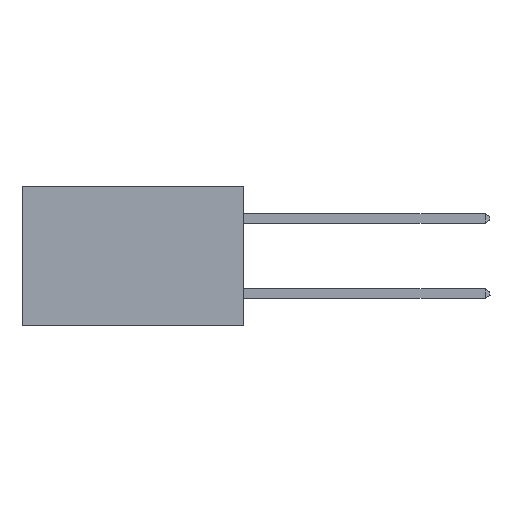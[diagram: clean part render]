
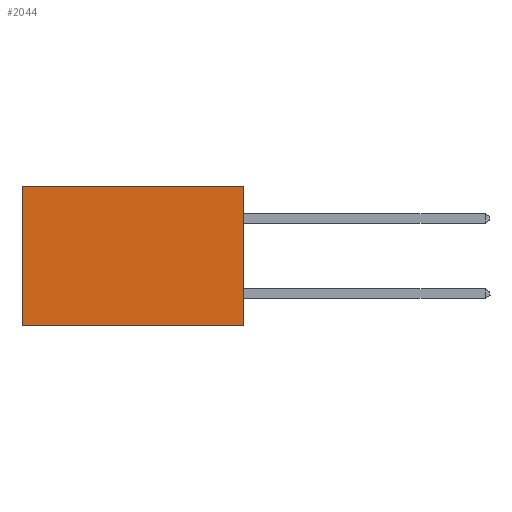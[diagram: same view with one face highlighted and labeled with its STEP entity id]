
A CAD part, left-side view. The second image highlights one B-rep face of the part: STEP entity #2044.
In plain terms, the highlighted planar face has unit normal (-1, 0, 0).
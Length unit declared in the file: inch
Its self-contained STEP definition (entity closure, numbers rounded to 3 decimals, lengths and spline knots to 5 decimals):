
#309 = CARTESIAN_POINT ( 'NONE',  ( 0.277, 0., 0. ) ) ;
#1711 = CARTESIAN_POINT ( 'NONE',  ( 0.277, 0.59, 0. ) ) ;
#2044 = ADVANCED_FACE ( 'NONE', ( #8573 ), #7231, .F. ) ;
#3269 = ORIENTED_EDGE ( 'NONE', *, *, #14440, .F. ) ;
#3280 = VERTEX_POINT ( 'NONE', #16151 ) ;
#4182 = VERTEX_POINT ( 'NONE', #17679 ) ;
#4478 = VECTOR ( 'NONE', #14712, 39.37008 ) ;
#4995 = EDGE_CURVE ( 'NONE', #7809, #6947, #7499, .T. ) ;
#6272 = LINE ( 'NONE', #16073, #9992 ) ;
#6947 = VERTEX_POINT ( 'NONE', #1711 ) ;
#7231 = PLANE ( 'NONE',  #7263 ) ;
#7255 = DIRECTION ( 'NONE',  ( 1., 0., 0. ) ) ;
#7263 = AXIS2_PLACEMENT_3D ( 'NONE', #13273, #7255, #14982 ) ;
#7499 = LINE ( 'NONE', #14310, #15017 ) ;
#7540 = EDGE_CURVE ( 'NONE', #7809, #4182, #8625, .T. ) ;
#7809 = VERTEX_POINT ( 'NONE', #309 ) ;
#8573 = FACE_OUTER_BOUND ( 'NONE', #17480, .T. ) ;
#8625 = LINE ( 'NONE', #14395, #4478 ) ;
#8811 = ORIENTED_EDGE ( 'NONE', *, *, #7540, .F. ) ;
#9992 = VECTOR ( 'NONE', #17835, 39.37008 ) ;
#10317 = LINE ( 'NONE', #17713, #13757 ) ;
#11874 = DIRECTION ( 'NONE',  ( 0., 0., -1. ) ) ;
#12437 = EDGE_CURVE ( 'NONE', #6947, #3280, #10317, .T. ) ;
#12860 = ORIENTED_EDGE ( 'NONE', *, *, #4995, .T. ) ;
#13273 = CARTESIAN_POINT ( 'NONE',  ( 0.277, 0., -0.37 ) ) ;
#13757 = VECTOR ( 'NONE', #11874, 39.37008 ) ;
#14310 = CARTESIAN_POINT ( 'NONE',  ( 0.277, 0., 0. ) ) ;
#14395 = CARTESIAN_POINT ( 'NONE',  ( 0.277, 0., -0.37 ) ) ;
#14440 = EDGE_CURVE ( 'NONE', #4182, #3280, #6272, .T. ) ;
#14712 = DIRECTION ( 'NONE',  ( 0., 0., -1. ) ) ;
#14982 = DIRECTION ( 'NONE',  ( 0., 0., -1. ) ) ;
#15017 = VECTOR ( 'NONE', #16835, 39.37008 ) ;
#15790 = ORIENTED_EDGE ( 'NONE', *, *, #12437, .T. ) ;
#16073 = CARTESIAN_POINT ( 'NONE',  ( 0.277, 0., -0.37 ) ) ;
#16151 = CARTESIAN_POINT ( 'NONE',  ( 0.277, 0.59, -0.37 ) ) ;
#16835 = DIRECTION ( 'NONE',  ( 0., 1., 0. ) ) ;
#17480 = EDGE_LOOP ( 'NONE', ( #15790, #3269, #8811, #12860 ) ) ;
#17679 = CARTESIAN_POINT ( 'NONE',  ( 0.277, 0., -0.37 ) ) ;
#17713 = CARTESIAN_POINT ( 'NONE',  ( 0.277, 0.59, -0.37 ) ) ;
#17835 = DIRECTION ( 'NONE',  ( 0., 1., 0. ) ) ;
